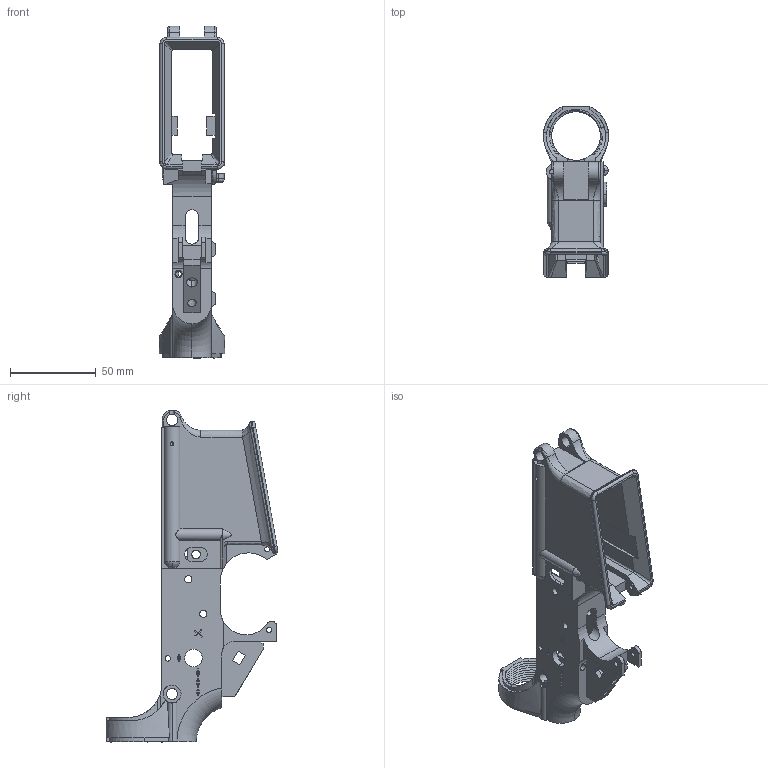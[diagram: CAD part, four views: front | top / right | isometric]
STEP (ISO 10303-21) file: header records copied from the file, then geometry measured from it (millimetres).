
FILE_DESCRIPTION (( 'STEP AP203' ), '1' );
FILE_NAME ('xr15_lower.STEP', '2021-12-29T04:22:09', ( '' ), ( '' ), 'SwSTEP 2.0', 'SolidWorks 2015', '' );
FILE_SCHEMA (( 'CONFIG_CONTROL_DESIGN' ));
Length unit declared in the file: millimetre
Products named in the file (1): xr15_lower
Bounding box: 38.11 x 100.05 x 193.8 mm (x, y, z)
Volume: 86117.3 mm3; surface area: 53988.7 mm2
Topology: 1 solids, 1 shells, 637 faces, 1818 edges, 1185 vertices
Faces by surface type: plane 369, cylinder 137, bspline 115, torus 11, sphere 4, cone 1
Entity records: 35856 total; most frequent: CARTESIAN_POINT 20051, ORIENTED_EDGE 3636, DIRECTION 2773, EDGE_CURVE 1818, VERTEX_POINT 1185, LINE 1137, VECTOR 1137, AXIS2_PLACEMENT_3D 818
